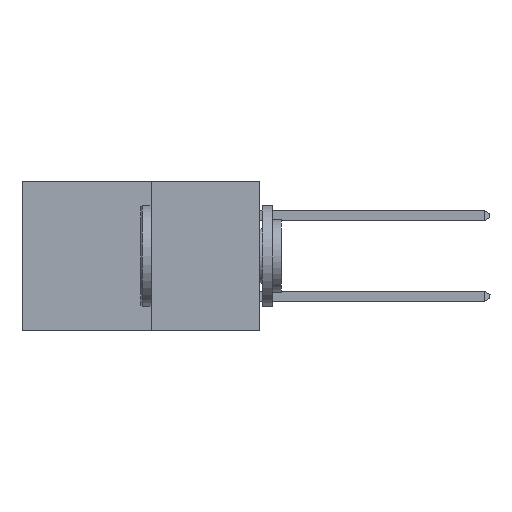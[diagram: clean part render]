
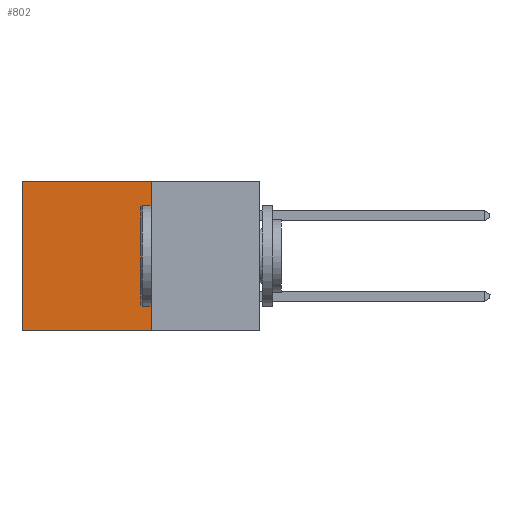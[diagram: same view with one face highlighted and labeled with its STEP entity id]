
A CAD part, left-side view. The second image highlights one B-rep face of the part: STEP entity #802.
In plain terms, the highlighted planar face has unit normal (-1, 0, 0).
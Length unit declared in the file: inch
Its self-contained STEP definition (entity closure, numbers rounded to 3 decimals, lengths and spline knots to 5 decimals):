
#152 = CARTESIAN_POINT ( 'NONE',  ( 0.277, 0.59, -0.37 ) ) ;
#499 = EDGE_CURVE ( 'NONE', #5088, #10250, #935, .T. ) ;
#694 = CARTESIAN_POINT ( 'NONE',  ( 0.277, 0.27, -0.37 ) ) ;
#802 = ADVANCED_FACE ( 'NONE', ( #2265 ), #1478, .F. ) ;
#935 = LINE ( 'NONE', #6282, #5386 ) ;
#1128 = LINE ( 'NONE', #6520, #9847 ) ;
#1246 = EDGE_CURVE ( 'NONE', #4104, #5088, #1508, .T. ) ;
#1478 = PLANE ( 'NONE',  #9209 ) ;
#1508 = LINE ( 'NONE', #694, #8069 ) ;
#2265 = FACE_OUTER_BOUND ( 'NONE', #7837, .T. ) ;
#3963 = CARTESIAN_POINT ( 'NONE',  ( 0.277, 0.59, 0. ) ) ;
#4104 = VERTEX_POINT ( 'NONE', #7351 ) ;
#4882 = ORIENTED_EDGE ( 'NONE', *, *, #10931, .T. ) ;
#5088 = VERTEX_POINT ( 'NONE', #10584 ) ;
#5243 = LINE ( 'NONE', #9937, #7219 ) ;
#5386 = VECTOR ( 'NONE', #6608, 39.37008 ) ;
#5633 = CARTESIAN_POINT ( 'NONE',  ( 0.277, 0.27, -0.37 ) ) ;
#5685 = ORIENTED_EDGE ( 'NONE', *, *, #1246, .F. ) ;
#5893 = DIRECTION ( 'NONE',  ( 0., 0., -1. ) ) ;
#5895 = ORIENTED_EDGE ( 'NONE', *, *, #499, .F. ) ;
#6123 = ORIENTED_EDGE ( 'NONE', *, *, #6362, .T. ) ;
#6282 = CARTESIAN_POINT ( 'NONE',  ( 0.277, 0.27, -0.37 ) ) ;
#6362 = EDGE_CURVE ( 'NONE', #9013, #10250, #5243, .T. ) ;
#6520 = CARTESIAN_POINT ( 'NONE',  ( 0.277, 0.27, 0. ) ) ;
#6608 = DIRECTION ( 'NONE',  ( 0., 1., 0. ) ) ;
#6799 = DIRECTION ( 'NONE',  ( 0., 0., -1. ) ) ;
#6869 = DIRECTION ( 'NONE',  ( 1., 0., 0. ) ) ;
#7219 = VECTOR ( 'NONE', #6799, 39.37008 ) ;
#7351 = CARTESIAN_POINT ( 'NONE',  ( 0.277, 0.27, 0. ) ) ;
#7354 = DIRECTION ( 'NONE',  ( 0., 1., 0. ) ) ;
#7488 = DIRECTION ( 'NONE',  ( 0., 0., -1. ) ) ;
#7837 = EDGE_LOOP ( 'NONE', ( #6123, #5895, #5685, #4882 ) ) ;
#8069 = VECTOR ( 'NONE', #7488, 39.37008 ) ;
#9013 = VERTEX_POINT ( 'NONE', #3963 ) ;
#9209 = AXIS2_PLACEMENT_3D ( 'NONE', #5633, #6869, #5893 ) ;
#9847 = VECTOR ( 'NONE', #7354, 39.37008 ) ;
#9937 = CARTESIAN_POINT ( 'NONE',  ( 0.277, 0.59, -0.37 ) ) ;
#10250 = VERTEX_POINT ( 'NONE', #152 ) ;
#10584 = CARTESIAN_POINT ( 'NONE',  ( 0.277, 0.27, -0.37 ) ) ;
#10931 = EDGE_CURVE ( 'NONE', #4104, #9013, #1128, .T. ) ;
